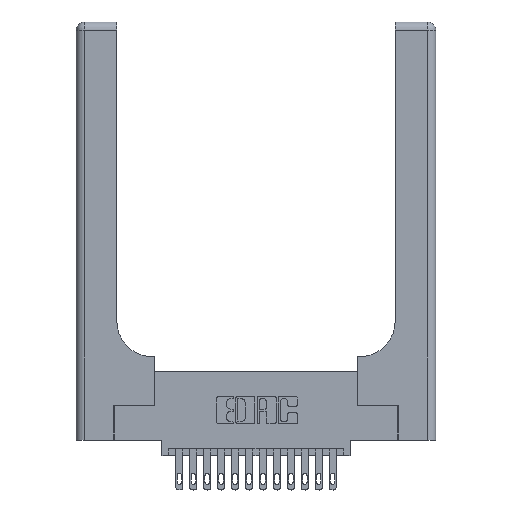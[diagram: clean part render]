
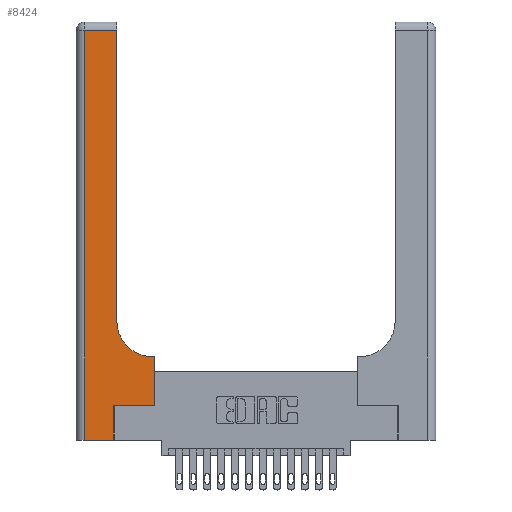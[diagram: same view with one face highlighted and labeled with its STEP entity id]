
A CAD part, top view. The second image highlights one B-rep face of the part: STEP entity #8424.
In plain terms, the highlighted planar face has unit normal (0, 0, 1).
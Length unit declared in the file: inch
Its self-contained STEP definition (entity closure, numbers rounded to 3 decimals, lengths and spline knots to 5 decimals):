
#178 = VECTOR ( 'NONE', #509, 39.37008 ) ;
#509 = DIRECTION ( 'NONE',  ( 0., -1., 0. ) ) ;
#711 = EDGE_CURVE ( 'NONE', #15775, #4298, #17055, .T. ) ;
#1075 = EDGE_CURVE ( 'NONE', #15753, #14430, #1728, .T. ) ;
#1215 = DIRECTION ( 'NONE',  ( 1., 0., 0. ) ) ;
#1575 = DIRECTION ( 'NONE',  ( 1., 0., 0. ) ) ;
#1728 = LINE ( 'NONE', #2701, #8926 ) ;
#2330 = ORIENTED_EDGE ( 'NONE', *, *, #5235, .T. ) ;
#2539 = CARTESIAN_POINT ( 'NONE',  ( 0.2915, 2.94, 0.37 ) ) ;
#2701 = CARTESIAN_POINT ( 'NONE',  ( 0.269, 0., 0.37 ) ) ;
#2755 = EDGE_LOOP ( 'NONE', ( #17358, #2330, #17479, #8711, #13021, #9350, #7423, #8619, #13644 ) ) ;
#2980 = CARTESIAN_POINT ( 'NONE',  ( 0., 2.94, 0.37 ) ) ;
#3512 = CARTESIAN_POINT ( 'NONE',  ( 0.5415, 0.6, 0.37 ) ) ;
#3525 = AXIS2_PLACEMENT_3D ( 'NONE', #7311, #7193, #9976 ) ;
#3959 = DIRECTION ( 'NONE',  ( 0., 1., 0. ) ) ;
#3993 = LINE ( 'NONE', #15579, #5311 ) ;
#4298 = VERTEX_POINT ( 'NONE', #3512 ) ;
#4321 = CARTESIAN_POINT ( 'NONE',  ( 0.5585, 0.25, 0.37 ) ) ;
#4417 = VERTEX_POINT ( 'NONE', #2539 ) ;
#4551 = EDGE_CURVE ( 'NONE', #4298, #10417, #6491, .T. ) ;
#4765 = VECTOR ( 'NONE', #1575, 39.37008 ) ;
#4768 = EDGE_CURVE ( 'NONE', #10594, #9266, #13039, .T. ) ;
#5235 = EDGE_CURVE ( 'NONE', #4417, #10594, #13482, .T. ) ;
#5311 = VECTOR ( 'NONE', #8393, 39.37008 ) ;
#5338 = DIRECTION ( 'NONE',  ( 0., 0., -1. ) ) ;
#5561 = VECTOR ( 'NONE', #6279, 39.37008 ) ;
#6279 = DIRECTION ( 'NONE',  ( -1., 0., 0. ) ) ;
#6408 = VERTEX_POINT ( 'NONE', #13146 ) ;
#6491 = CIRCLE ( 'NONE', #3525, 0.25 ) ;
#7028 = EDGE_CURVE ( 'NONE', #10417, #4417, #3993, .T. ) ;
#7193 = DIRECTION ( 'NONE',  ( 0., 0., -1. ) ) ;
#7237 = CARTESIAN_POINT ( 'NONE',  ( 0.269, 0., 0.37 ) ) ;
#7311 = CARTESIAN_POINT ( 'NONE',  ( 0.5415, 0.85, 0.37 ) ) ;
#7423 = ORIENTED_EDGE ( 'NONE', *, *, #15671, .T. ) ;
#7698 = CARTESIAN_POINT ( 'NONE',  ( 0.5585, 0.6, 0.37 ) ) ;
#8383 = LINE ( 'NONE', #9860, #11527 ) ;
#8393 = DIRECTION ( 'NONE',  ( 0., 1., 0. ) ) ;
#8424 = ADVANCED_FACE ( 'NONE', ( #18389 ), #18599, .F. ) ;
#8579 = LINE ( 'NONE', #14036, #4765 ) ;
#8619 = ORIENTED_EDGE ( 'NONE', *, *, #711, .T. ) ;
#8711 = ORIENTED_EDGE ( 'NONE', *, *, #17623, .T. ) ;
#8926 = VECTOR ( 'NONE', #17225, 39.37008 ) ;
#8986 = DIRECTION ( 'NONE',  ( -1., 0., 0. ) ) ;
#9266 = VERTEX_POINT ( 'NONE', #18440 ) ;
#9350 = ORIENTED_EDGE ( 'NONE', *, *, #16532, .T. ) ;
#9420 = CARTESIAN_POINT ( 'NONE',  ( 0.2915, 0.6, 0.37 ) ) ;
#9860 = CARTESIAN_POINT ( 'NONE',  ( 0.269, 0.25, 0.37 ) ) ;
#9976 = DIRECTION ( 'NONE',  ( 1., 0., 0. ) ) ;
#10111 = VECTOR ( 'NONE', #8986, 39.37008 ) ;
#10417 = VERTEX_POINT ( 'NONE', #11043 ) ;
#10594 = VERTEX_POINT ( 'NONE', #15829 ) ;
#11043 = CARTESIAN_POINT ( 'NONE',  ( 0.2915, 0.85, 0.37 ) ) ;
#11527 = VECTOR ( 'NONE', #1215, 39.37008 ) ;
#11750 = CARTESIAN_POINT ( 'NONE',  ( 0.269, 0.25, 0.37 ) ) ;
#12765 = CARTESIAN_POINT ( 'NONE',  ( 0., 3., 0.37 ) ) ;
#13021 = ORIENTED_EDGE ( 'NONE', *, *, #1075, .T. ) ;
#13039 = LINE ( 'NONE', #16193, #178 ) ;
#13146 = CARTESIAN_POINT ( 'NONE',  ( 0.5585, 0.25, 0.37 ) ) ;
#13482 = LINE ( 'NONE', #2980, #10111 ) ;
#13644 = ORIENTED_EDGE ( 'NONE', *, *, #4551, .T. ) ;
#14036 = CARTESIAN_POINT ( 'NONE',  ( 0., 0., 0.37 ) ) ;
#14037 = LINE ( 'NONE', #4321, #15404 ) ;
#14430 = VERTEX_POINT ( 'NONE', #11750 ) ;
#15404 = VECTOR ( 'NONE', #3959, 39.37008 ) ;
#15415 = DIRECTION ( 'NONE',  ( -1., 0., 0. ) ) ;
#15579 = CARTESIAN_POINT ( 'NONE',  ( 0.2915, 3., 0.37 ) ) ;
#15671 = EDGE_CURVE ( 'NONE', #6408, #15775, #14037, .T. ) ;
#15753 = VERTEX_POINT ( 'NONE', #7237 ) ;
#15775 = VERTEX_POINT ( 'NONE', #7698 ) ;
#15829 = CARTESIAN_POINT ( 'NONE',  ( 0.06, 2.94, 0.37 ) ) ;
#16193 = CARTESIAN_POINT ( 'NONE',  ( 0.06, 3., 0.37 ) ) ;
#16532 = EDGE_CURVE ( 'NONE', #14430, #6408, #8383, .T. ) ;
#17055 = LINE ( 'NONE', #9420, #5561 ) ;
#17225 = DIRECTION ( 'NONE',  ( 0., 1., 0. ) ) ;
#17358 = ORIENTED_EDGE ( 'NONE', *, *, #7028, .T. ) ;
#17479 = ORIENTED_EDGE ( 'NONE', *, *, #4768, .T. ) ;
#17623 = EDGE_CURVE ( 'NONE', #9266, #15753, #8579, .T. ) ;
#17660 = AXIS2_PLACEMENT_3D ( 'NONE', #12765, #5338, #15415 ) ;
#18389 = FACE_OUTER_BOUND ( 'NONE', #2755, .T. ) ;
#18440 = CARTESIAN_POINT ( 'NONE',  ( 0.06, 0., 0.37 ) ) ;
#18599 = PLANE ( 'NONE',  #17660 ) ;
